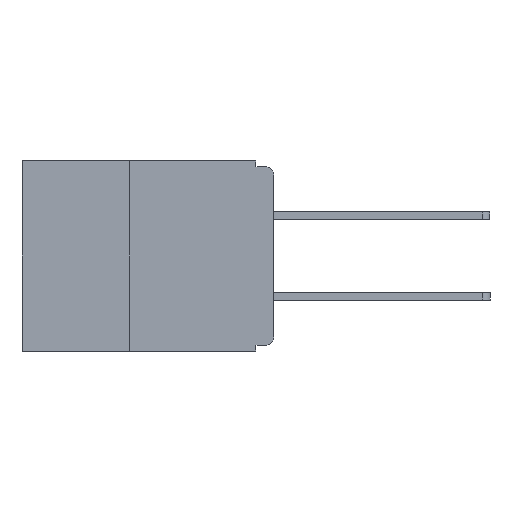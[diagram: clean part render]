
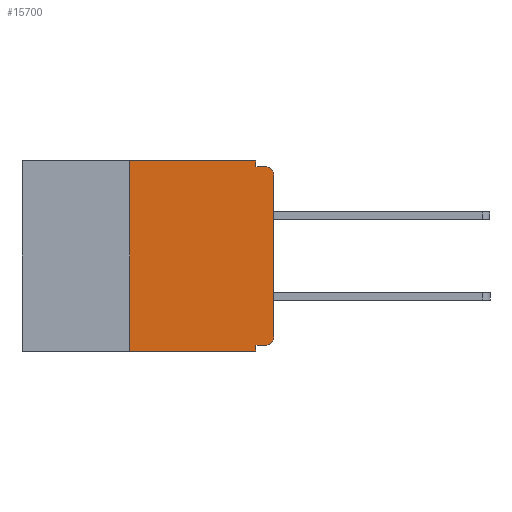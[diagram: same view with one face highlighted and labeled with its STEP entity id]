
A CAD part, left-side view. The second image highlights one B-rep face of the part: STEP entity #15700.
In plain terms, the highlighted planar face has unit normal (-1, 0, 0).
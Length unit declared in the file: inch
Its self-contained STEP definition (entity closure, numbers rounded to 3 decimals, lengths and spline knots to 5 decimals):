
#893 = DIRECTION ( 'NONE',  ( 1., 0., 0. ) ) ;
#1403 = EDGE_CURVE ( 'NONE', #23553, #16251, #10240, .T. ) ;
#1483 = ORIENTED_EDGE ( 'NONE', *, *, #15575, .T. ) ;
#2652 = EDGE_LOOP ( 'NONE', ( #20514, #20678, #5309, #5477, #14281, #18631, #12343, #17548, #7727, #1483 ) ) ;
#2657 = EDGE_CURVE ( 'NONE', #18014, #11009, #7850, .T. ) ;
#2786 = CARTESIAN_POINT ( 'NONE',  ( 0., 0., -0.025 ) ) ;
#2877 = EDGE_CURVE ( 'NONE', #17989, #18014, #18827, .T. ) ;
#4661 = AXIS2_PLACEMENT_3D ( 'NONE', #9166, #23898, #11312 ) ;
#4938 = AXIS2_PLACEMENT_3D ( 'NONE', #10507, #10477, #10437 ) ;
#4997 = LINE ( 'NONE', #23828, #6365 ) ;
#5309 = ORIENTED_EDGE ( 'NONE', *, *, #8332, .F. ) ;
#5467 = CARTESIAN_POINT ( 'NONE',  ( 0., 0.031, -0.01 ) ) ;
#5477 = ORIENTED_EDGE ( 'NONE', *, *, #16259, .F. ) ;
#5565 = VECTOR ( 'NONE', #25795, 39.37008 ) ;
#6365 = VECTOR ( 'NONE', #11257, 39.37008 ) ;
#6672 = LINE ( 'NONE', #23845, #11723 ) ;
#7257 = DIRECTION ( 'NONE',  ( 0., 0., -1. ) ) ;
#7727 = ORIENTED_EDGE ( 'NONE', *, *, #21081, .F. ) ;
#7850 = CIRCLE ( 'NONE', #4938, 0.015 ) ;
#8332 = EDGE_CURVE ( 'NONE', #10720, #11009, #26651, .T. ) ;
#9166 = CARTESIAN_POINT ( 'NONE',  ( 0., 0.015, -0.305 ) ) ;
#9287 = CARTESIAN_POINT ( 'NONE',  ( 0., 0.437, 0. ) ) ;
#9351 = VERTEX_POINT ( 'NONE', #20107 ) ;
#9405 = LINE ( 'NONE', #9287, #25517 ) ;
#10240 = LINE ( 'NONE', #10338, #26324 ) ;
#10338 = CARTESIAN_POINT ( 'NONE',  ( 0., 0.25, -0.33 ) ) ;
#10437 = DIRECTION ( 'NONE',  ( 0., 0., -1. ) ) ;
#10477 = DIRECTION ( 'NONE',  ( -1., 0., 0. ) ) ;
#10507 = CARTESIAN_POINT ( 'NONE',  ( 0., 0.015, -0.025 ) ) ;
#10720 = VERTEX_POINT ( 'NONE', #5467 ) ;
#11009 = VERTEX_POINT ( 'NONE', #25515 ) ;
#11140 = CARTESIAN_POINT ( 'NONE',  ( 0., 0.437, -0.33 ) ) ;
#11257 = DIRECTION ( 'NONE',  ( 0., 1., 0. ) ) ;
#11312 = DIRECTION ( 'NONE',  ( 0., 0., -1. ) ) ;
#11476 = CARTESIAN_POINT ( 'NONE',  ( 0., 0.25, 0. ) ) ;
#11610 = CIRCLE ( 'NONE', #4661, 0.015 ) ;
#11723 = VECTOR ( 'NONE', #26017, 39.37008 ) ;
#12028 = CARTESIAN_POINT ( 'NONE',  ( 0., 0.031, -0.33 ) ) ;
#12343 = ORIENTED_EDGE ( 'NONE', *, *, #20368, .T. ) ;
#12595 = FACE_OUTER_BOUND ( 'NONE', #2652, .T. ) ;
#13005 = EDGE_CURVE ( 'NONE', #19325, #19352, #6672, .T. ) ;
#13060 = CARTESIAN_POINT ( 'NONE',  ( 0., 0.015, -0.32 ) ) ;
#13240 = VECTOR ( 'NONE', #27046, 39.37008 ) ;
#13427 = VERTEX_POINT ( 'NONE', #13060 ) ;
#13966 = CARTESIAN_POINT ( 'NONE',  ( 0., 0.437, 0. ) ) ;
#14281 = ORIENTED_EDGE ( 'NONE', *, *, #21160, .F. ) ;
#15554 = VECTOR ( 'NONE', #7257, 39.37008 ) ;
#15575 = EDGE_CURVE ( 'NONE', #13427, #17989, #11610, .T. ) ;
#15700 = ADVANCED_FACE ( 'NONE', ( #12595 ), #22296, .F. ) ;
#16057 = DIRECTION ( 'NONE',  ( 0., 0., -1. ) ) ;
#16251 = VERTEX_POINT ( 'NONE', #11476 ) ;
#16259 = EDGE_CURVE ( 'NONE', #9351, #10720, #22454, .T. ) ;
#17548 = ORIENTED_EDGE ( 'NONE', *, *, #13005, .F. ) ;
#17989 = VERTEX_POINT ( 'NONE', #21877 ) ;
#18014 = VERTEX_POINT ( 'NONE', #2786 ) ;
#18631 = ORIENTED_EDGE ( 'NONE', *, *, #1403, .F. ) ;
#18827 = LINE ( 'NONE', #20772, #13240 ) ;
#19325 = VERTEX_POINT ( 'NONE', #24571 ) ;
#19352 = VERTEX_POINT ( 'NONE', #12028 ) ;
#19694 = DIRECTION ( 'NONE',  ( 0., -1., 0. ) ) ;
#19997 = CARTESIAN_POINT ( 'NONE',  ( 0., 0.031, 0. ) ) ;
#20107 = CARTESIAN_POINT ( 'NONE',  ( 0., 0.031, 0. ) ) ;
#20368 = EDGE_CURVE ( 'NONE', #23553, #19352, #27307, .T. ) ;
#20514 = ORIENTED_EDGE ( 'NONE', *, *, #2877, .T. ) ;
#20678 = ORIENTED_EDGE ( 'NONE', *, *, #2657, .T. ) ;
#20772 = CARTESIAN_POINT ( 'NONE',  ( 0., 0., 0. ) ) ;
#21081 = EDGE_CURVE ( 'NONE', #13427, #19325, #4997, .T. ) ;
#21160 = EDGE_CURVE ( 'NONE', #16251, #9351, #9405, .T. ) ;
#21195 = VECTOR ( 'NONE', #19694, 39.37008 ) ;
#21877 = CARTESIAN_POINT ( 'NONE',  ( 0., 0., -0.305 ) ) ;
#21957 = DIRECTION ( 'NONE',  ( 0., -1., 0. ) ) ;
#22296 = PLANE ( 'NONE',  #24552 ) ;
#22454 = LINE ( 'NONE', #19997, #15554 ) ;
#23553 = VERTEX_POINT ( 'NONE', #27321 ) ;
#23828 = CARTESIAN_POINT ( 'NONE',  ( 0., 0., -0.32 ) ) ;
#23845 = CARTESIAN_POINT ( 'NONE',  ( 0., 0.031, -0.33 ) ) ;
#23872 = DIRECTION ( 'NONE',  ( 0., 0., 1. ) ) ;
#23898 = DIRECTION ( 'NONE',  ( -1., 0., 0. ) ) ;
#24552 = AXIS2_PLACEMENT_3D ( 'NONE', #13966, #893, #16057 ) ;
#24571 = CARTESIAN_POINT ( 'NONE',  ( 0., 0.031, -0.32 ) ) ;
#25515 = CARTESIAN_POINT ( 'NONE',  ( 0., 0.015, -0.01 ) ) ;
#25517 = VECTOR ( 'NONE', #21957, 39.37008 ) ;
#25795 = DIRECTION ( 'NONE',  ( 0., -1., 0. ) ) ;
#25817 = CARTESIAN_POINT ( 'NONE',  ( 0., 0., -0.01 ) ) ;
#26017 = DIRECTION ( 'NONE',  ( 0., 0., -1. ) ) ;
#26324 = VECTOR ( 'NONE', #23872, 39.37008 ) ;
#26651 = LINE ( 'NONE', #25817, #21195 ) ;
#27046 = DIRECTION ( 'NONE',  ( 0., 0., 1. ) ) ;
#27307 = LINE ( 'NONE', #11140, #5565 ) ;
#27321 = CARTESIAN_POINT ( 'NONE',  ( 0., 0.25, -0.33 ) ) ;
